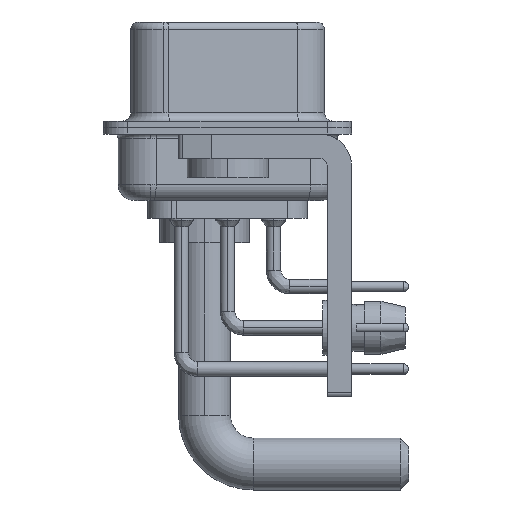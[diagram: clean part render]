
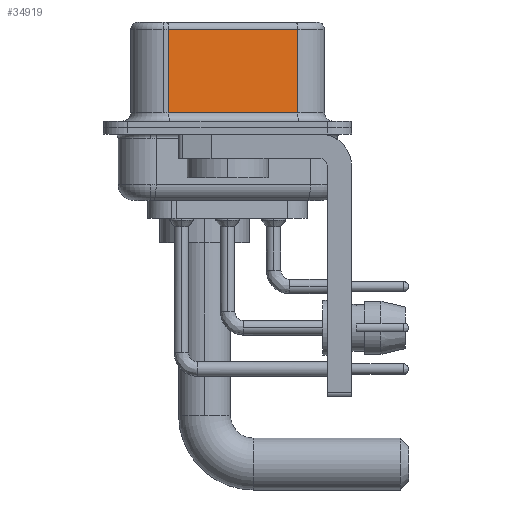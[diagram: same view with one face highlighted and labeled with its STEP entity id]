
A CAD part, left-side view. The second image highlights one B-rep face of the part: STEP entity #34919.
In plain terms, the highlighted planar face has unit normal (-0.985, -0.174, 0).
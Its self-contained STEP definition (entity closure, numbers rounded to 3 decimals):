
#821 = ORIENTED_EDGE ( 'NONE', *, *, #7041, .T. ) ;
#2227 = LINE ( 'NONE', #7511, #32785 ) ;
#4056 = CARTESIAN_POINT ( 'NONE',  ( 5.132, -4.322, 6.02 ) ) ;
#6357 = EDGE_CURVE ( 'NONE', #27279, #27382, #9580, .T. ) ;
#7041 = EDGE_CURVE ( 'NONE', #32111, #27279, #20981, .T. ) ;
#7511 = CARTESIAN_POINT ( 'NONE',  ( 5.132, -4.322, 0.9 ) ) ;
#9417 = CARTESIAN_POINT ( 'NONE',  ( 3.73, 3.628, 0.9 ) ) ;
#9580 = LINE ( 'NONE', #27783, #15205 ) ;
#11717 = VECTOR ( 'NONE', #27258, 1000. ) ;
#12170 = ORIENTED_EDGE ( 'NONE', *, *, #6357, .T. ) ;
#14159 = AXIS2_PLACEMENT_3D ( 'NONE', #38557, #38768, #22999 ) ;
#15205 = VECTOR ( 'NONE', #34245, 1000. ) ;
#17543 = PLANE ( 'NONE',  #14159 ) ;
#17891 = EDGE_CURVE ( 'NONE', #27382, #19809, #2227, .T. ) ;
#19054 = EDGE_LOOP ( 'NONE', ( #21789, #821, #12170, #28790 ) ) ;
#19809 = VERTEX_POINT ( 'NONE', #31717 ) ;
#20807 = CARTESIAN_POINT ( 'NONE',  ( 5.132, -4.322, 6.52 ) ) ;
#20981 = LINE ( 'NONE', #21594, #32399 ) ;
#21594 = CARTESIAN_POINT ( 'NONE',  ( 5.132, -4.322, 6.02 ) ) ;
#21789 = ORIENTED_EDGE ( 'NONE', *, *, #26778, .F. ) ;
#22999 = DIRECTION ( 'NONE',  ( -0.174, 0.985, 0. ) ) ;
#23197 = FACE_OUTER_BOUND ( 'NONE', #19054, .T. ) ;
#26778 = EDGE_CURVE ( 'NONE', #32111, #19809, #39791, .T. ) ;
#27207 = CARTESIAN_POINT ( 'NONE',  ( 3.73, 3.628, 6.02 ) ) ;
#27258 = DIRECTION ( 'NONE',  ( 0., 0., -1. ) ) ;
#27279 = VERTEX_POINT ( 'NONE', #27207 ) ;
#27382 = VERTEX_POINT ( 'NONE', #9417 ) ;
#27783 = CARTESIAN_POINT ( 'NONE',  ( 3.73, 3.628, 6.52 ) ) ;
#28790 = ORIENTED_EDGE ( 'NONE', *, *, #17891, .T. ) ;
#31717 = CARTESIAN_POINT ( 'NONE',  ( 5.132, -4.322, 0.9 ) ) ;
#32111 = VERTEX_POINT ( 'NONE', #4056 ) ;
#32399 = VECTOR ( 'NONE', #33499, 1000. ) ;
#32785 = VECTOR ( 'NONE', #38429, 1000. ) ;
#33499 = DIRECTION ( 'NONE',  ( -0.174, 0.985, 0. ) ) ;
#34245 = DIRECTION ( 'NONE',  ( 0., 0., -1. ) ) ;
#34919 = ADVANCED_FACE ( 'NONE', ( #23197 ), #17543, .F. ) ;
#38429 = DIRECTION ( 'NONE',  ( 0.174, -0.985, 0. ) ) ;
#38557 = CARTESIAN_POINT ( 'NONE',  ( 5.132, -4.322, 6.52 ) ) ;
#38768 = DIRECTION ( 'NONE',  ( 0.985, 0.174, 0. ) ) ;
#39791 = LINE ( 'NONE', #20807, #11717 ) ;
